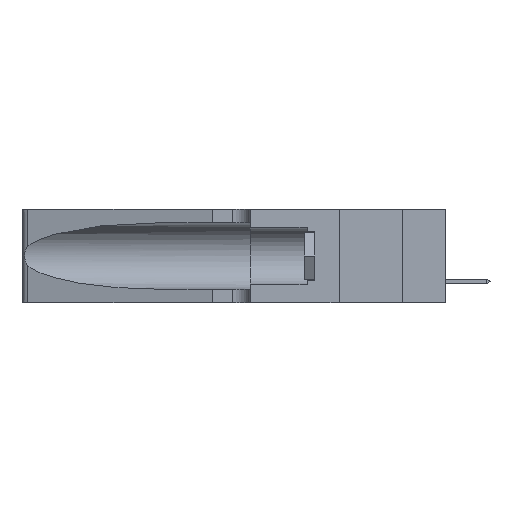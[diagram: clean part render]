
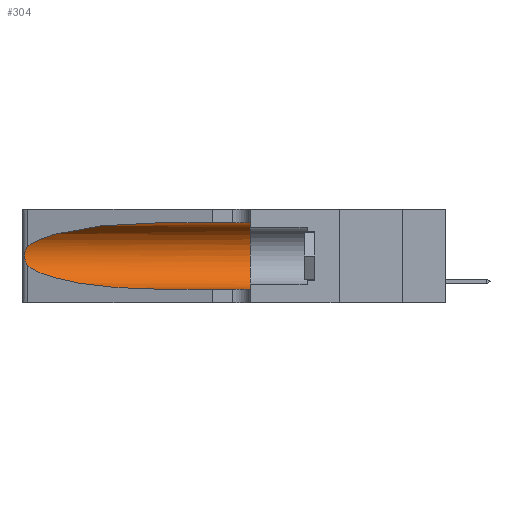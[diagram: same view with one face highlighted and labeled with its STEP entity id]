
A CAD part, left-side view. The second image highlights one B-rep face of the part: STEP entity #304.
In plain terms, the highlighted cylindrical face has radius 3.308 mm (diameter 6.617 mm), a partial arc.
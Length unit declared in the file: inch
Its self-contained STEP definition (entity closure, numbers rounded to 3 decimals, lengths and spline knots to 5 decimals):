
#304 = ADVANCED_FACE ( 'NONE', ( #26091 ), #5525, .F. ) ;
#942 = AXIS2_PLACEMENT_3D ( 'NONE', #25146, #8546, #13151 ) ;
#2019 = CARTESIAN_POINT ( 'NONE',  ( 0.18966, 0.96281, 0.31525 ) ) ;
#2283 = VERTEX_POINT ( 'NONE', #10223 ) ;
#4602 = CARTESIAN_POINT ( 'NONE',  ( 0.26075, 1.23896, 0.178 ) ) ;
#4804 = CARTESIAN_POINT ( 'NONE',  ( 0.25856, 1.23593, 0.16098 ) ) ;
#4926 = DIRECTION ( 'NONE',  ( 0., -1., 0. ) ) ;
#5247 = VECTOR ( 'NONE', #4926, 39.37008 ) ;
#5346 = CARTESIAN_POINT ( 'NONE',  ( 0.18966, 0.96281, 0.05475 ) ) ;
#5525 = CYLINDRICAL_SURFACE ( 'NONE', #30152, 0.13025 ) ;
#5738 = ORIENTED_EDGE ( 'NONE', *, *, #26610, .T. ) ;
#5806 = DIRECTION ( 'NONE',  ( 0., -1., 0. ) ) ;
#7109 = LINE ( 'NONE', #14325, #5247 ) ;
#7214 = CARTESIAN_POINT ( 'NONE',  ( 0.25854, 1.2359, 0.20912 ) ) ;
#7655 = CARTESIAN_POINT ( 'NONE',  ( 0.1305, 1.61858, 0.31525 ) ) ;
#7763 = CARTESIAN_POINT ( 'NONE',  ( 0.2373, 1.15595, 0.08982 ) ) ;
#8211 = VECTOR ( 'NONE', #15276, 39.37008 ) ;
#8357 = ORIENTED_EDGE ( 'NONE', *, *, #16445, .F. ) ;
#8546 = DIRECTION ( 'NONE',  ( 0., 1., 0. ) ) ;
#8777 =( BOUNDED_CURVE ( )  B_SPLINE_CURVE ( 3, ( #11300, #2019, #11615, #26050 ),
 .UNSPECIFIED., .F., .F. ) 
 B_SPLINE_CURVE_WITH_KNOTS ( ( 4, 4 ),
 ( 1.5708, 2.84003 ),
 .UNSPECIFIED. ) 
 CURVE ( )  GEOMETRIC_REPRESENTATION_ITEM ( )  RATIONAL_B_SPLINE_CURVE ( ( 1., 0.87, 0.87, 1. ) ) 
 REPRESENTATION_ITEM ( '' )  );
#9327 = CARTESIAN_POINT ( 'NONE',  ( 0.1305, 0.72297, 0.05475 ) ) ;
#9338 =( BOUNDED_CURVE ( )  B_SPLINE_CURVE ( 3, ( #12325, #7763, #5346, #24445 ),
 .UNSPECIFIED., .F., .F. ) 
 B_SPLINE_CURVE_WITH_KNOTS ( ( 4, 4 ),
 ( 3.44316, 4.71239 ),
 .UNSPECIFIED. ) 
 CURVE ( )  GEOMETRIC_REPRESENTATION_ITEM ( )  RATIONAL_B_SPLINE_CURVE ( ( 1., 0.87, 0.87, 1. ) ) 
 REPRESENTATION_ITEM ( '' )  );
#9517 = CARTESIAN_POINT ( 'NONE',  ( 0.26017, 1.23833, 0.17102 ) ) ;
#9819 = ORIENTED_EDGE ( 'NONE', *, *, #30637, .F. ) ;
#10223 = CARTESIAN_POINT ( 'NONE',  ( 0.1305, 0.72297, 0.31525 ) ) ;
#10505 = CARTESIAN_POINT ( 'NONE',  ( 0.1305, 1.61858, 0.185 ) ) ;
#10765 = EDGE_CURVE ( 'NONE', #18130, #18374, #13290, .T. ) ;
#10817 = CARTESIAN_POINT ( 'NONE',  ( 0.1305, 0.35, 0.05475 ) ) ;
#11300 = CARTESIAN_POINT ( 'NONE',  ( 0.1305, 0.72297, 0.31525 ) ) ;
#11615 = CARTESIAN_POINT ( 'NONE',  ( 0.2373, 1.15595, 0.28018 ) ) ;
#11878 = CARTESIAN_POINT ( 'NONE',  ( 0.25555, 1.22993, 0.14849 ) ) ;
#12325 = CARTESIAN_POINT ( 'NONE',  ( 0.25487, 1.22718, 0.14631 ) ) ;
#13151 = DIRECTION ( 'NONE',  ( 0., 0., 1. ) ) ;
#13290 = B_SPLINE_CURVE_WITH_KNOTS ( 'NONE', 3,
 ( #14402, #14204, #16696, #30908, #7214, #16595, #21407, #4602, #9517, #4804, #21299, #21506, #11878, #28624 ),
 .UNSPECIFIED., .F., .F.,
 ( 4, 2, 2, 2, 2, 2, 4 ),
 ( 0., 0.00027, 0.00053, 0.00107, 0.0016, 0.00187, 0.00214 ),
 .UNSPECIFIED. ) ;
#14132 = CIRCLE ( 'NONE', #942, 0.13025 ) ;
#14204 = CARTESIAN_POINT ( 'NONE',  ( 0.25555, 1.22994, 0.2215 ) ) ;
#14325 = CARTESIAN_POINT ( 'NONE',  ( 0.1305, 1.61858, 0.05475 ) ) ;
#14394 = CARTESIAN_POINT ( 'NONE',  ( 0.25487, 1.22718, 0.14631 ) ) ;
#14402 = CARTESIAN_POINT ( 'NONE',  ( 0.25487, 1.22718, 0.22369 ) ) ;
#15041 = VERTEX_POINT ( 'NONE', #29606 ) ;
#15276 = DIRECTION ( 'NONE',  ( 0., -1., 0. ) ) ;
#16426 = VERTEX_POINT ( 'NONE', #10817 ) ;
#16445 = EDGE_CURVE ( 'NONE', #15041, #16426, #14132, .T. ) ;
#16595 = CARTESIAN_POINT ( 'NONE',  ( 0.26018, 1.23835, 0.19895 ) ) ;
#16696 = CARTESIAN_POINT ( 'NONE',  ( 0.25639, 1.23184, 0.21858 ) ) ;
#17811 = EDGE_CURVE ( 'NONE', #18374, #19544, #9338, .T. ) ;
#18130 = VERTEX_POINT ( 'NONE', #23799 ) ;
#18374 = VERTEX_POINT ( 'NONE', #14394 ) ;
#19544 = VERTEX_POINT ( 'NONE', #9327 ) ;
#20313 = ORIENTED_EDGE ( 'NONE', *, *, #10765, .T. ) ;
#21299 = CARTESIAN_POINT ( 'NONE',  ( 0.25789, 1.23486, 0.15765 ) ) ;
#21407 = CARTESIAN_POINT ( 'NONE',  ( 0.26075, 1.23896, 0.19203 ) ) ;
#21506 = CARTESIAN_POINT ( 'NONE',  ( 0.25639, 1.23186, 0.15144 ) ) ;
#22313 = EDGE_CURVE ( 'NONE', #19544, #16426, #7109, .T. ) ;
#23799 = CARTESIAN_POINT ( 'NONE',  ( 0.25487, 1.22718, 0.22369 ) ) ;
#24445 = CARTESIAN_POINT ( 'NONE',  ( 0.1305, 0.72297, 0.05475 ) ) ;
#25146 = CARTESIAN_POINT ( 'NONE',  ( 0.1305, 0.35, 0.185 ) ) ;
#25147 = ORIENTED_EDGE ( 'NONE', *, *, #17811, .T. ) ;
#26050 = CARTESIAN_POINT ( 'NONE',  ( 0.25487, 1.22718, 0.22369 ) ) ;
#26091 = FACE_OUTER_BOUND ( 'NONE', #28251, .T. ) ;
#26610 = EDGE_CURVE ( 'NONE', #2283, #18130, #8777, .T. ) ;
#27262 = LINE ( 'NONE', #7655, #8211 ) ;
#27330 = DIRECTION ( 'NONE',  ( 0., 0., -1. ) ) ;
#28251 = EDGE_LOOP ( 'NONE', ( #5738, #20313, #25147, #28509, #8357, #9819 ) ) ;
#28509 = ORIENTED_EDGE ( 'NONE', *, *, #22313, .T. ) ;
#28624 = CARTESIAN_POINT ( 'NONE',  ( 0.25487, 1.22718, 0.14631 ) ) ;
#29606 = CARTESIAN_POINT ( 'NONE',  ( 0.1305, 0.35, 0.31525 ) ) ;
#30152 = AXIS2_PLACEMENT_3D ( 'NONE', #10505, #5806, #27330 ) ;
#30637 = EDGE_CURVE ( 'NONE', #2283, #15041, #27262, .T. ) ;
#30908 = CARTESIAN_POINT ( 'NONE',  ( 0.25787, 1.23484, 0.2124 ) ) ;
